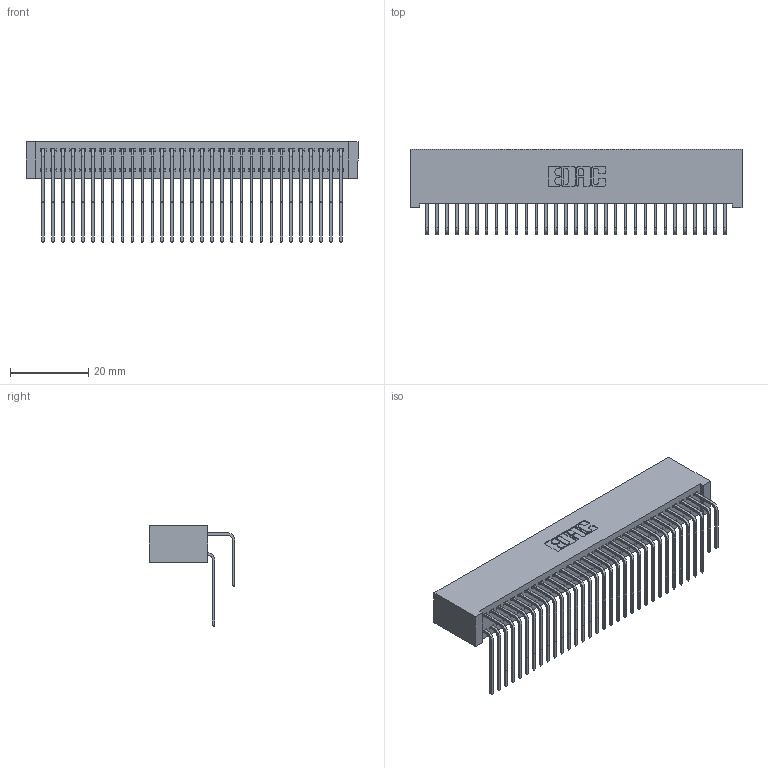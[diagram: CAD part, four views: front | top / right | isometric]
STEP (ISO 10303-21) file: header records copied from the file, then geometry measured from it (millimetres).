
FILE_DESCRIPTION (( 'STEP AP203' ), '1' );
FILE_NAME ('342-062-558-201.STEP', '2018-08-13T06:58:13', ( '' ), ( '' ), 'SwSTEP 2.0', 'SolidWorks 2016', '' );
FILE_SCHEMA (( 'CONFIG_CONTROL_DESIGN' ));
Length unit declared in the file: inch
Products named in the file (4): 342 Part_Lugless; 345-292-001_558 559 Tail - 1; 345-292-001_558 Tail - 2; 342-062-558-201
Assembly tree (63 placements, depth 2):
  342-062-558-201
    342 Part_Lugless
    345-292-001_558 559 Tail - 1  x31
    345-292-001_558 Tail - 2  x31
Bounding box: 84.99 x 21.91 x 25.78 mm (x, y, z)
Volume: 8381.3 mm3; surface area: 15435.8 mm2
Topology: 63 solids, 63 shells, 3450 faces, 10257 edges, 6754 vertices
Faces by surface type: plane 2418, cylinder 1032
Entity records: 22741 total; most frequent: CARTESIAN_POINT 3829, ORIENTED_EDGE 3714, DIRECTION 3265, EDGE_CURVE 1857, LINE 1697, VECTOR 1697, VERTEX_POINT 1234, AXIS2_PLACEMENT_3D 784
